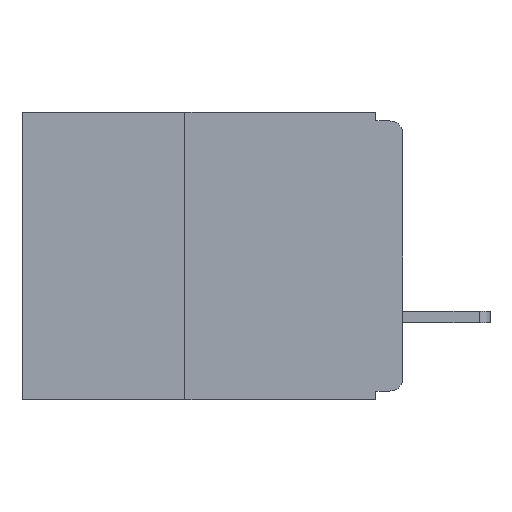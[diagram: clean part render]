
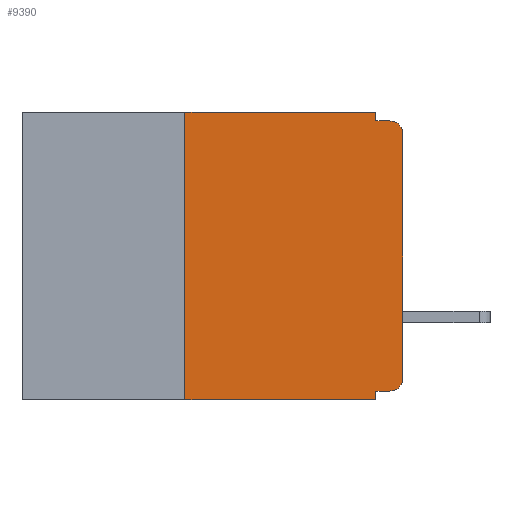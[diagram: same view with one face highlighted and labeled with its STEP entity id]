
A CAD part, left-side view. The second image highlights one B-rep face of the part: STEP entity #9390.
In plain terms, the highlighted planar face has unit normal (-1, 0, 0).
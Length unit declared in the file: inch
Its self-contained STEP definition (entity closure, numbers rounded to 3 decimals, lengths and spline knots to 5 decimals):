
#70 = DIRECTION ( 'NONE',  ( -1., 0., 0. ) ) ;
#351 = CARTESIAN_POINT ( 'NONE',  ( 0., 0.031, -0.01 ) ) ;
#356 = VERTEX_POINT ( 'NONE', #11861 ) ;
#589 = EDGE_CURVE ( 'NONE', #22413, #17010, #15423, .T. ) ;
#594 = CARTESIAN_POINT ( 'NONE',  ( 0., 0.437, 0. ) ) ;
#1216 = DIRECTION ( 'NONE',  ( 0., -1., 0. ) ) ;
#1297 = EDGE_CURVE ( 'NONE', #12263, #13705, #4398, .T. ) ;
#1675 = EDGE_CURVE ( 'NONE', #12263, #356, #10659, .T. ) ;
#1686 = CARTESIAN_POINT ( 'NONE',  ( 0., 0.25, -0.33 ) ) ;
#1840 = CARTESIAN_POINT ( 'NONE',  ( 0., 0.437, -0.33 ) ) ;
#2132 = ORIENTED_EDGE ( 'NONE', *, *, #589, .F. ) ;
#2478 = DIRECTION ( 'NONE',  ( 1., 0., 0. ) ) ;
#2697 = ORIENTED_EDGE ( 'NONE', *, *, #12524, .T. ) ;
#2861 = DIRECTION ( 'NONE',  ( 0., -1., 0. ) ) ;
#3031 = DIRECTION ( 'NONE',  ( 0., 0., 1. ) ) ;
#3240 = ORIENTED_EDGE ( 'NONE', *, *, #18827, .F. ) ;
#3547 = VECTOR ( 'NONE', #3031, 39.37008 ) ;
#4122 = CARTESIAN_POINT ( 'NONE',  ( 0., 0.015, -0.32 ) ) ;
#4398 = CIRCLE ( 'NONE', #20952, 0.015 ) ;
#4730 = CARTESIAN_POINT ( 'NONE',  ( 0., 0., -0.025 ) ) ;
#4814 = VECTOR ( 'NONE', #1216, 39.37008 ) ;
#4964 = LINE ( 'NONE', #15311, #10686 ) ;
#5404 = LINE ( 'NONE', #20351, #19867 ) ;
#5625 = EDGE_CURVE ( 'NONE', #21592, #13193, #14961, .T. ) ;
#5785 = EDGE_CURVE ( 'NONE', #356, #6775, #7291, .T. ) ;
#5829 = VERTEX_POINT ( 'NONE', #4730 ) ;
#6177 = CARTESIAN_POINT ( 'NONE',  ( 0., 0.437, 0. ) ) ;
#6299 = ORIENTED_EDGE ( 'NONE', *, *, #12102, .T. ) ;
#6775 = VERTEX_POINT ( 'NONE', #18505 ) ;
#7291 = LINE ( 'NONE', #9757, #21623 ) ;
#7476 = CARTESIAN_POINT ( 'NONE',  ( 0., 0.015, -0.025 ) ) ;
#8210 = CARTESIAN_POINT ( 'NONE',  ( 0., 0., -0.32 ) ) ;
#9039 = ORIENTED_EDGE ( 'NONE', *, *, #5625, .F. ) ;
#9390 = ADVANCED_FACE ( 'NONE', ( #13615 ), #13831, .F. ) ;
#9423 = DIRECTION ( 'NONE',  ( 0., 0., -1. ) ) ;
#9757 = CARTESIAN_POINT ( 'NONE',  ( 0., 0.031, -0.33 ) ) ;
#9807 = VERTEX_POINT ( 'NONE', #1686 ) ;
#9957 = ORIENTED_EDGE ( 'NONE', *, *, #1297, .T. ) ;
#9995 = CARTESIAN_POINT ( 'NONE',  ( 0., 0., -0.01 ) ) ;
#10137 = ORIENTED_EDGE ( 'NONE', *, *, #1675, .F. ) ;
#10659 = LINE ( 'NONE', #8210, #21140 ) ;
#10686 = VECTOR ( 'NONE', #17179, 39.37008 ) ;
#11861 = CARTESIAN_POINT ( 'NONE',  ( 0., 0.031, -0.32 ) ) ;
#12102 = EDGE_CURVE ( 'NONE', #5829, #17010, #21797, .T. ) ;
#12263 = VERTEX_POINT ( 'NONE', #4122 ) ;
#12524 = EDGE_CURVE ( 'NONE', #13705, #5829, #13675, .T. ) ;
#12647 = EDGE_LOOP ( 'NONE', ( #2697, #6299, #2132, #3240, #9039, #21935, #23391, #20242, #10137, #9957 ) ) ;
#12941 = LINE ( 'NONE', #1840, #17325 ) ;
#13138 = CARTESIAN_POINT ( 'NONE',  ( 0., 0.031, 0. ) ) ;
#13193 = VERTEX_POINT ( 'NONE', #13138 ) ;
#13615 = FACE_OUTER_BOUND ( 'NONE', #12647, .T. ) ;
#13675 = LINE ( 'NONE', #23621, #3547 ) ;
#13705 = VERTEX_POINT ( 'NONE', #22407 ) ;
#13831 = PLANE ( 'NONE',  #15240 ) ;
#14961 = LINE ( 'NONE', #594, #4814 ) ;
#15240 = AXIS2_PLACEMENT_3D ( 'NONE', #6177, #2478, #15720 ) ;
#15311 = CARTESIAN_POINT ( 'NONE',  ( 0., 0.031, 0. ) ) ;
#15423 = LINE ( 'NONE', #9995, #19753 ) ;
#15720 = DIRECTION ( 'NONE',  ( 0., 0., -1. ) ) ;
#16079 = EDGE_CURVE ( 'NONE', #9807, #21592, #5404, .T. ) ;
#16977 = DIRECTION ( 'NONE',  ( 0., -1., 0. ) ) ;
#17010 = VERTEX_POINT ( 'NONE', #24280 ) ;
#17131 = DIRECTION ( 'NONE',  ( 0., 1., 0. ) ) ;
#17179 = DIRECTION ( 'NONE',  ( 0., 0., -1. ) ) ;
#17325 = VECTOR ( 'NONE', #16977, 39.37008 ) ;
#17329 = AXIS2_PLACEMENT_3D ( 'NONE', #7476, #20554, #9423 ) ;
#18505 = CARTESIAN_POINT ( 'NONE',  ( 0., 0.031, -0.33 ) ) ;
#18827 = EDGE_CURVE ( 'NONE', #13193, #22413, #4964, .T. ) ;
#19753 = VECTOR ( 'NONE', #2861, 39.37008 ) ;
#19867 = VECTOR ( 'NONE', #20431, 39.37008 ) ;
#20242 = ORIENTED_EDGE ( 'NONE', *, *, #5785, .F. ) ;
#20351 = CARTESIAN_POINT ( 'NONE',  ( 0., 0.25, -0.33 ) ) ;
#20431 = DIRECTION ( 'NONE',  ( 0., 0., 1. ) ) ;
#20554 = DIRECTION ( 'NONE',  ( -1., 0., 0. ) ) ;
#20952 = AXIS2_PLACEMENT_3D ( 'NONE', #22411, #70, #23445 ) ;
#21140 = VECTOR ( 'NONE', #17131, 39.37008 ) ;
#21198 = EDGE_CURVE ( 'NONE', #9807, #6775, #12941, .T. ) ;
#21381 = DIRECTION ( 'NONE',  ( 0., 0., -1. ) ) ;
#21592 = VERTEX_POINT ( 'NONE', #23646 ) ;
#21623 = VECTOR ( 'NONE', #21381, 39.37008 ) ;
#21797 = CIRCLE ( 'NONE', #17329, 0.015 ) ;
#21935 = ORIENTED_EDGE ( 'NONE', *, *, #16079, .F. ) ;
#22407 = CARTESIAN_POINT ( 'NONE',  ( 0., 0., -0.305 ) ) ;
#22411 = CARTESIAN_POINT ( 'NONE',  ( 0., 0.015, -0.305 ) ) ;
#22413 = VERTEX_POINT ( 'NONE', #351 ) ;
#23391 = ORIENTED_EDGE ( 'NONE', *, *, #21198, .T. ) ;
#23445 = DIRECTION ( 'NONE',  ( 0., 0., -1. ) ) ;
#23621 = CARTESIAN_POINT ( 'NONE',  ( 0., 0., 0. ) ) ;
#23646 = CARTESIAN_POINT ( 'NONE',  ( 0., 0.25, 0. ) ) ;
#24280 = CARTESIAN_POINT ( 'NONE',  ( 0., 0.015, -0.01 ) ) ;
